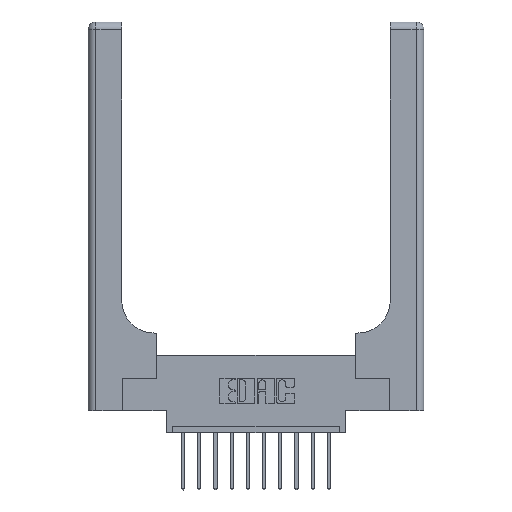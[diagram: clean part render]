
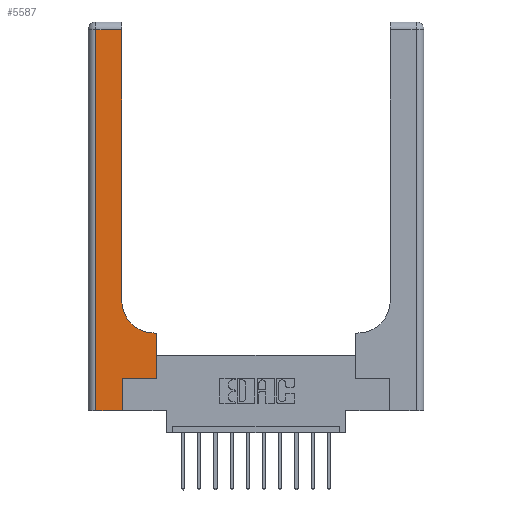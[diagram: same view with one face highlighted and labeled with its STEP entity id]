
A CAD part, top view. The second image highlights one B-rep face of the part: STEP entity #5587.
In plain terms, the highlighted planar face has unit normal (0, 0, 1).
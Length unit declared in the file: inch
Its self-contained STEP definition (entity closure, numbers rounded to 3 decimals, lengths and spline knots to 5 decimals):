
#53 = PLANE ( 'NONE',  #5254 ) ;
#131 = CARTESIAN_POINT ( 'NONE',  ( 0.26, 3., 0.37 ) ) ;
#146 = DIRECTION ( 'NONE',  ( 0., 0., -1. ) ) ;
#596 = LINE ( 'NONE', #8086, #10376 ) ;
#1459 = CARTESIAN_POINT ( 'NONE',  ( 0.06, 0., 0.37 ) ) ;
#1474 = DIRECTION ( 'NONE',  ( 0., 0., -1. ) ) ;
#1480 = ORIENTED_EDGE ( 'NONE', *, *, #8817, .T. ) ;
#1555 = CARTESIAN_POINT ( 'NONE',  ( 0.06, 3., 0.37 ) ) ;
#1667 = DIRECTION ( 'NONE',  ( -1., 0., 0. ) ) ;
#1727 = FACE_OUTER_BOUND ( 'NONE', #7016, .T. ) ;
#1969 = DIRECTION ( 'NONE',  ( 0., 1., 0. ) ) ;
#2110 = VECTOR ( 'NONE', #1969, 39.37008 ) ;
#2370 = EDGE_CURVE ( 'NONE', #14902, #11173, #15441, .T. ) ;
#2776 = EDGE_CURVE ( 'NONE', #10749, #5643, #5841, .T. ) ;
#3062 = EDGE_CURVE ( 'NONE', #9333, #14902, #11191, .T. ) ;
#3273 = CARTESIAN_POINT ( 'NONE',  ( 0., 0., 0.37 ) ) ;
#3453 = CARTESIAN_POINT ( 'NONE',  ( 0.528, 0.6, 0.37 ) ) ;
#3560 = EDGE_CURVE ( 'NONE', #4368, #15812, #14243, .T. ) ;
#4228 = CARTESIAN_POINT ( 'NONE',  ( 0.265, 0.25, 0.37 ) ) ;
#4368 = VERTEX_POINT ( 'NONE', #12749 ) ;
#4553 = CARTESIAN_POINT ( 'NONE',  ( 0.265, 0., 0.37 ) ) ;
#4652 = ORIENTED_EDGE ( 'NONE', *, *, #3062, .T. ) ;
#5103 = LINE ( 'NONE', #3273, #8770 ) ;
#5137 = VERTEX_POINT ( 'NONE', #1459 ) ;
#5207 = EDGE_CURVE ( 'NONE', #5643, #5137, #8273, .T. ) ;
#5254 = AXIS2_PLACEMENT_3D ( 'NONE', #8614, #146, #14825 ) ;
#5587 = ADVANCED_FACE ( 'NONE', ( #1727 ), #53, .F. ) ;
#5643 = VERTEX_POINT ( 'NONE', #12173 ) ;
#5841 = LINE ( 'NONE', #10108, #6617 ) ;
#5928 = ORIENTED_EDGE ( 'NONE', *, *, #14692, .T. ) ;
#6049 = ORIENTED_EDGE ( 'NONE', *, *, #5207, .T. ) ;
#6111 = DIRECTION ( 'NONE',  ( 0., 1., 0. ) ) ;
#6617 = VECTOR ( 'NONE', #1667, 39.37008 ) ;
#6813 = DIRECTION ( 'NONE',  ( 1., 0., 0. ) ) ;
#7016 = EDGE_LOOP ( 'NONE', ( #5928, #11637, #6049, #1480, #11886, #15786, #8338, #4652, #9884 ) ) ;
#7068 = VECTOR ( 'NONE', #6111, 39.37008 ) ;
#8078 = VERTEX_POINT ( 'NONE', #9781 ) ;
#8086 = CARTESIAN_POINT ( 'NONE',  ( 0.528, 0.25, 0.37 ) ) ;
#8273 = LINE ( 'NONE', #1555, #14395 ) ;
#8338 = ORIENTED_EDGE ( 'NONE', *, *, #12481, .T. ) ;
#8614 = CARTESIAN_POINT ( 'NONE',  ( 0., 3., 0.37 ) ) ;
#8770 = VECTOR ( 'NONE', #6813, 39.37008 ) ;
#8817 = EDGE_CURVE ( 'NONE', #5137, #4368, #5103, .T. ) ;
#8883 = CARTESIAN_POINT ( 'NONE',  ( 0.265, 0.25, 0.37 ) ) ;
#9333 = VERTEX_POINT ( 'NONE', #3453 ) ;
#9612 = CARTESIAN_POINT ( 'NONE',  ( 0.26, 2.94, 0.37 ) ) ;
#9619 = CARTESIAN_POINT ( 'NONE',  ( 0.26, 0.6, 0.37 ) ) ;
#9781 = CARTESIAN_POINT ( 'NONE',  ( 0.528, 0.25, 0.37 ) ) ;
#9884 = ORIENTED_EDGE ( 'NONE', *, *, #2370, .T. ) ;
#10041 = VECTOR ( 'NONE', #14545, 39.37008 ) ;
#10108 = CARTESIAN_POINT ( 'NONE',  ( 0., 2.94, 0.37 ) ) ;
#10126 = LINE ( 'NONE', #131, #7068 ) ;
#10219 = DIRECTION ( 'NONE',  ( 0., -1., 0. ) ) ;
#10376 = VECTOR ( 'NONE', #12370, 39.37008 ) ;
#10749 = VERTEX_POINT ( 'NONE', #9612 ) ;
#11173 = VERTEX_POINT ( 'NONE', #15858 ) ;
#11191 = LINE ( 'NONE', #9619, #10041 ) ;
#11292 = VECTOR ( 'NONE', #15214, 39.37008 ) ;
#11383 = AXIS2_PLACEMENT_3D ( 'NONE', #13931, #1474, #12623 ) ;
#11637 = ORIENTED_EDGE ( 'NONE', *, *, #2776, .T. ) ;
#11886 = ORIENTED_EDGE ( 'NONE', *, *, #3560, .T. ) ;
#12173 = CARTESIAN_POINT ( 'NONE',  ( 0.06, 2.94, 0.37 ) ) ;
#12370 = DIRECTION ( 'NONE',  ( 0., 1., 0. ) ) ;
#12481 = EDGE_CURVE ( 'NONE', #8078, #9333, #596, .T. ) ;
#12623 = DIRECTION ( 'NONE',  ( 1., 0., 0. ) ) ;
#12749 = CARTESIAN_POINT ( 'NONE',  ( 0.265, 0., 0.37 ) ) ;
#13711 = EDGE_CURVE ( 'NONE', #15812, #8078, #14941, .T. ) ;
#13931 = CARTESIAN_POINT ( 'NONE',  ( 0.51, 0.85, 0.37 ) ) ;
#14243 = LINE ( 'NONE', #4553, #2110 ) ;
#14395 = VECTOR ( 'NONE', #10219, 39.37008 ) ;
#14545 = DIRECTION ( 'NONE',  ( -1., 0., 0. ) ) ;
#14692 = EDGE_CURVE ( 'NONE', #11173, #10749, #10126, .T. ) ;
#14825 = DIRECTION ( 'NONE',  ( -1., 0., 0. ) ) ;
#14902 = VERTEX_POINT ( 'NONE', #15372 ) ;
#14941 = LINE ( 'NONE', #4228, #11292 ) ;
#15214 = DIRECTION ( 'NONE',  ( 1., 0., 0. ) ) ;
#15372 = CARTESIAN_POINT ( 'NONE',  ( 0.51, 0.6, 0.37 ) ) ;
#15441 = CIRCLE ( 'NONE', #11383, 0.25 ) ;
#15786 = ORIENTED_EDGE ( 'NONE', *, *, #13711, .T. ) ;
#15812 = VERTEX_POINT ( 'NONE', #8883 ) ;
#15858 = CARTESIAN_POINT ( 'NONE',  ( 0.26, 0.85, 0.37 ) ) ;
